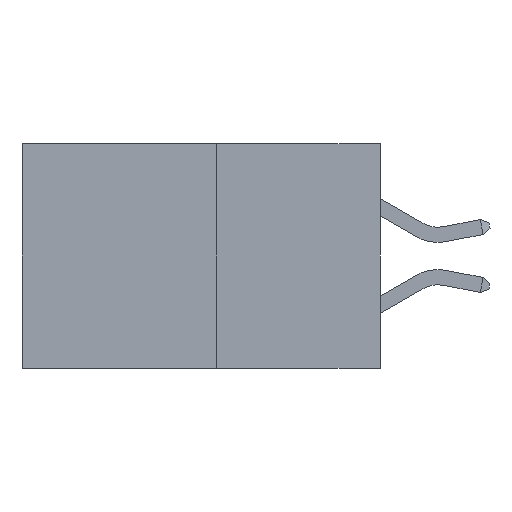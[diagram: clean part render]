
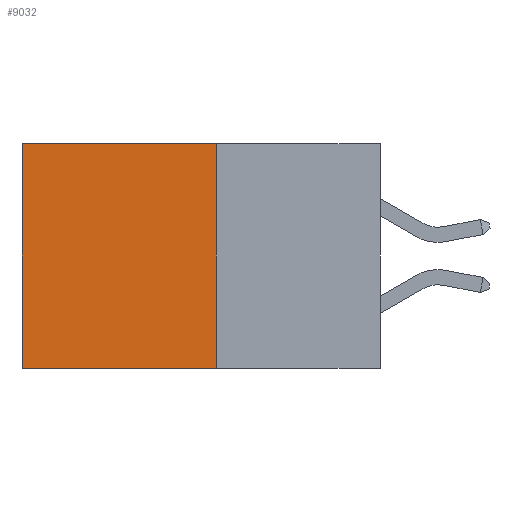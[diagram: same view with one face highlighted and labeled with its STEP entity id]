
A CAD part, left-side view. The second image highlights one B-rep face of the part: STEP entity #9032.
In plain terms, the highlighted planar face has unit normal (-1, 0, 0).
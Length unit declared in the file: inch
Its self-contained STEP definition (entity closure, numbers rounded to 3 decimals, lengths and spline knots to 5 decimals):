
#264 = VERTEX_POINT ( 'NONE', #3485 ) ;
#299 = DIRECTION ( 'NONE',  ( 0., 1., 0. ) ) ;
#727 = AXIS2_PLACEMENT_3D ( 'NONE', #5948, #3844, #8834 ) ;
#917 = DIRECTION ( 'NONE',  ( 0., 1., 0. ) ) ;
#1857 = VERTEX_POINT ( 'NONE', #6863 ) ;
#1938 = EDGE_LOOP ( 'NONE', ( #7658, #4991, #5656, #4223 ) ) ;
#2016 = LINE ( 'NONE', #5233, #7495 ) ;
#2141 = VECTOR ( 'NONE', #3546, 39.37008 ) ;
#2747 = VECTOR ( 'NONE', #299, 39.37008 ) ;
#2815 = CARTESIAN_POINT ( 'NONE',  ( 0.277, 0.27, -0.37 ) ) ;
#3123 = PLANE ( 'NONE',  #727 ) ;
#3461 = CARTESIAN_POINT ( 'NONE',  ( 0.277, 0.27, -0.37 ) ) ;
#3485 = CARTESIAN_POINT ( 'NONE',  ( 0.277, 0.59, 0. ) ) ;
#3546 = DIRECTION ( 'NONE',  ( 0., 0., -1. ) ) ;
#3844 = DIRECTION ( 'NONE',  ( 1., 0., 0. ) ) ;
#3907 = CARTESIAN_POINT ( 'NONE',  ( 0.277, 0.27, -0.37 ) ) ;
#4223 = ORIENTED_EDGE ( 'NONE', *, *, #8986, .T. ) ;
#4446 = EDGE_CURVE ( 'NONE', #264, #1857, #9054, .T. ) ;
#4875 = LINE ( 'NONE', #3907, #2747 ) ;
#4991 = ORIENTED_EDGE ( 'NONE', *, *, #7280, .F. ) ;
#5233 = CARTESIAN_POINT ( 'NONE',  ( 0.277, 0.27, 0. ) ) ;
#5282 = VECTOR ( 'NONE', #7891, 39.37008 ) ;
#5656 = ORIENTED_EDGE ( 'NONE', *, *, #8747, .F. ) ;
#5948 = CARTESIAN_POINT ( 'NONE',  ( 0.277, 0.27, -0.37 ) ) ;
#6863 = CARTESIAN_POINT ( 'NONE',  ( 0.277, 0.59, -0.37 ) ) ;
#7021 = FACE_OUTER_BOUND ( 'NONE', #1938, .T. ) ;
#7280 = EDGE_CURVE ( 'NONE', #8031, #1857, #4875, .T. ) ;
#7360 = VERTEX_POINT ( 'NONE', #8268 ) ;
#7495 = VECTOR ( 'NONE', #917, 39.37008 ) ;
#7604 = LINE ( 'NONE', #2815, #2141 ) ;
#7658 = ORIENTED_EDGE ( 'NONE', *, *, #4446, .T. ) ;
#7891 = DIRECTION ( 'NONE',  ( 0., 0., -1. ) ) ;
#8031 = VERTEX_POINT ( 'NONE', #3461 ) ;
#8268 = CARTESIAN_POINT ( 'NONE',  ( 0.277, 0.27, 0. ) ) ;
#8747 = EDGE_CURVE ( 'NONE', #7360, #8031, #7604, .T. ) ;
#8834 = DIRECTION ( 'NONE',  ( 0., 0., -1. ) ) ;
#8986 = EDGE_CURVE ( 'NONE', #7360, #264, #2016, .T. ) ;
#9032 = ADVANCED_FACE ( 'NONE', ( #7021 ), #3123, .F. ) ;
#9054 = LINE ( 'NONE', #9287, #5282 ) ;
#9287 = CARTESIAN_POINT ( 'NONE',  ( 0.277, 0.59, -0.37 ) ) ;
